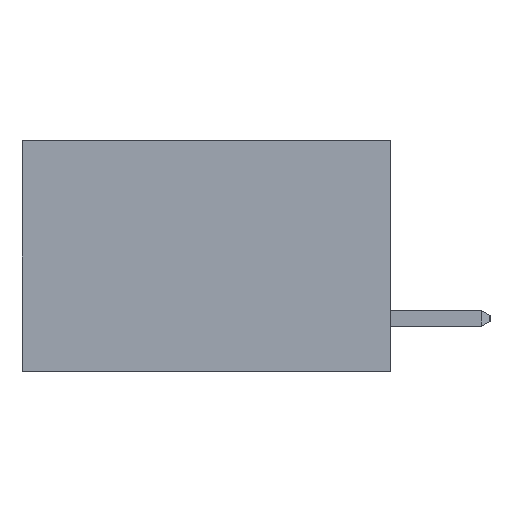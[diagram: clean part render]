
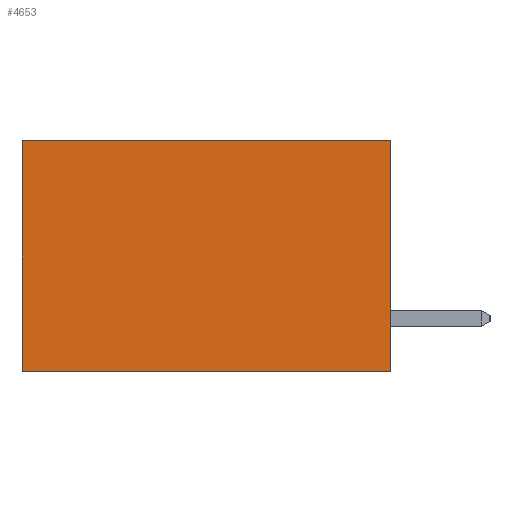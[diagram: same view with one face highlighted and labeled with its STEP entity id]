
A CAD part, left-side view. The second image highlights one B-rep face of the part: STEP entity #4653.
In plain terms, the highlighted planar face has unit normal (-1, 0, 0).
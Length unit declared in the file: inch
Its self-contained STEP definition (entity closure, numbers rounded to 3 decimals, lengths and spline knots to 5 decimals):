
#112 = VECTOR ( 'NONE', #1031, 39.37008 ) ;
#187 = EDGE_CURVE ( 'NONE', #1988, #5499, #7491, .T. ) ;
#413 = VERTEX_POINT ( 'NONE', #1324 ) ;
#1031 = DIRECTION ( 'NONE',  ( 0., 0., -1. ) ) ;
#1324 = CARTESIAN_POINT ( 'NONE',  ( 0.277, 0., 0. ) ) ;
#1367 = PLANE ( 'NONE',  #6672 ) ;
#1371 = DIRECTION ( 'NONE',  ( 0., 0., -1. ) ) ;
#1407 = DIRECTION ( 'NONE',  ( 1., 0., 0. ) ) ;
#1468 = CARTESIAN_POINT ( 'NONE',  ( 0.277, 0., -0.37 ) ) ;
#1568 = DIRECTION ( 'NONE',  ( 0., 1., 0. ) ) ;
#1894 = CARTESIAN_POINT ( 'NONE',  ( 0.277, 0., -0.37 ) ) ;
#1988 = VERTEX_POINT ( 'NONE', #4792 ) ;
#2018 = VECTOR ( 'NONE', #17293, 39.37008 ) ;
#2240 = ORIENTED_EDGE ( 'NONE', *, *, #15742, .T. ) ;
#2304 = DIRECTION ( 'NONE',  ( 0., 0., -1. ) ) ;
#2790 = FACE_OUTER_BOUND ( 'NONE', #3644, .T. ) ;
#3644 = EDGE_LOOP ( 'NONE', ( #12263, #10363, #13110, #2240 ) ) ;
#3857 = CARTESIAN_POINT ( 'NONE',  ( 0.277, 0., -0.37 ) ) ;
#4653 = ADVANCED_FACE ( 'NONE', ( #2790 ), #1367, .F. ) ;
#4792 = CARTESIAN_POINT ( 'NONE',  ( 0.277, 0.59, 0. ) ) ;
#5499 = VERTEX_POINT ( 'NONE', #8088 ) ;
#5746 = VERTEX_POINT ( 'NONE', #3857 ) ;
#5828 = EDGE_CURVE ( 'NONE', #413, #5746, #9197, .T. ) ;
#6110 = LINE ( 'NONE', #8413, #9276 ) ;
#6566 = CARTESIAN_POINT ( 'NONE',  ( 0.277, 0., 0. ) ) ;
#6672 = AXIS2_PLACEMENT_3D ( 'NONE', #1468, #1407, #1371 ) ;
#7491 = LINE ( 'NONE', #15911, #112 ) ;
#8088 = CARTESIAN_POINT ( 'NONE',  ( 0.277, 0.59, -0.37 ) ) ;
#8413 = CARTESIAN_POINT ( 'NONE',  ( 0.277, 0., -0.37 ) ) ;
#9197 = LINE ( 'NONE', #1894, #15896 ) ;
#9276 = VECTOR ( 'NONE', #1568, 39.37008 ) ;
#9459 = EDGE_CURVE ( 'NONE', #5746, #5499, #6110, .T. ) ;
#10363 = ORIENTED_EDGE ( 'NONE', *, *, #9459, .F. ) ;
#12263 = ORIENTED_EDGE ( 'NONE', *, *, #187, .T. ) ;
#13110 = ORIENTED_EDGE ( 'NONE', *, *, #5828, .F. ) ;
#15742 = EDGE_CURVE ( 'NONE', #413, #1988, #16025, .T. ) ;
#15896 = VECTOR ( 'NONE', #2304, 39.37008 ) ;
#15911 = CARTESIAN_POINT ( 'NONE',  ( 0.277, 0.59, -0.37 ) ) ;
#16025 = LINE ( 'NONE', #6566, #2018 ) ;
#17293 = DIRECTION ( 'NONE',  ( 0., 1., 0. ) ) ;
